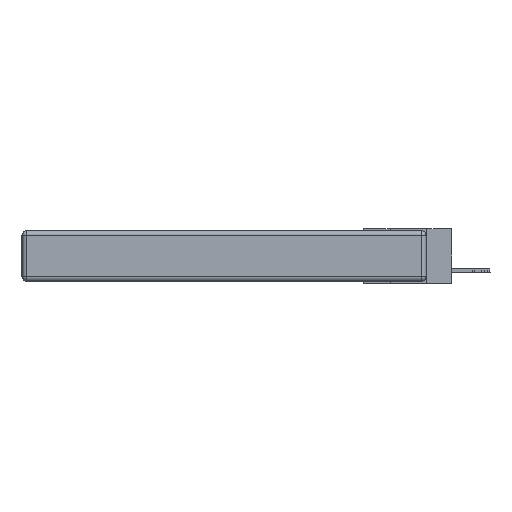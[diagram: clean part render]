
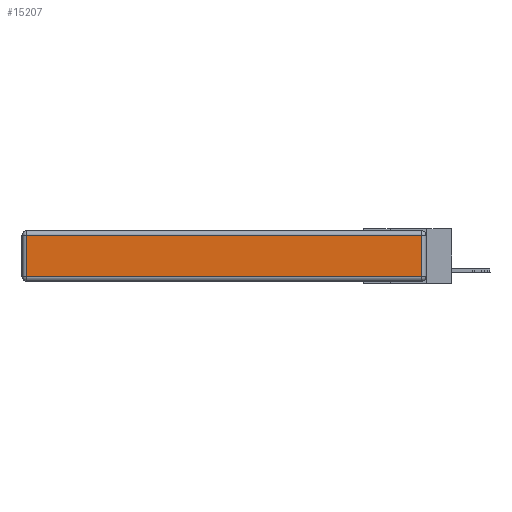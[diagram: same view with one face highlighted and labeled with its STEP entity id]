
A CAD part, left-side view. The second image highlights one B-rep face of the part: STEP entity #15207.
In plain terms, the highlighted planar face has unit normal (-1, 0, 0).
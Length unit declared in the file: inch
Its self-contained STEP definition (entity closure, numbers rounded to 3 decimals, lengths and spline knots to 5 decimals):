
#182 = ORIENTED_EDGE ( 'NONE', *, *, #19351, .T. ) ;
#227 = VERTEX_POINT ( 'NONE', #25936 ) ;
#235 = CARTESIAN_POINT ( 'NONE',  ( 0., 0.03, -0.343 ) ) ;
#1325 = PLANE ( 'NONE',  #10417 ) ;
#2420 = DIRECTION ( 'NONE',  ( 0., 0., 1. ) ) ;
#5226 = VECTOR ( 'NONE', #2420, 39.37008 ) ;
#6656 = DIRECTION ( 'NONE',  ( 0., 0., 1. ) ) ;
#8117 = CARTESIAN_POINT ( 'NONE',  ( 0., 0., -0.313 ) ) ;
#8878 = FACE_OUTER_BOUND ( 'NONE', #27182, .T. ) ;
#10362 = ORIENTED_EDGE ( 'NONE', *, *, #26238, .T. ) ;
#10417 = AXIS2_PLACEMENT_3D ( 'NONE', #11458, #18902, #6656 ) ;
#11458 = CARTESIAN_POINT ( 'NONE',  ( 0., 0., -0.343 ) ) ;
#12166 = VERTEX_POINT ( 'NONE', #22477 ) ;
#13234 = LINE ( 'NONE', #8117, #27146 ) ;
#13450 = VECTOR ( 'NONE', #22171, 39.37008 ) ;
#14374 = VECTOR ( 'NONE', #28630, 39.37008 ) ;
#15207 = ADVANCED_FACE ( 'NONE', ( #8878 ), #1325, .T. ) ;
#15752 = LINE ( 'NONE', #235, #5226 ) ;
#18863 = CARTESIAN_POINT ( 'NONE',  ( 0., 0.03, -0.313 ) ) ;
#18902 = DIRECTION ( 'NONE',  ( -1., 0., 0. ) ) ;
#19351 = EDGE_CURVE ( 'NONE', #31159, #12166, #20966, .T. ) ;
#20891 = CARTESIAN_POINT ( 'NONE',  ( 0., 2.72, -0.343 ) ) ;
#20966 = LINE ( 'NONE', #20891, #14374 ) ;
#21743 = EDGE_CURVE ( 'NONE', #22734, #227, #15752, .T. ) ;
#22171 = DIRECTION ( 'NONE',  ( 0., 1., 0. ) ) ;
#22279 = CARTESIAN_POINT ( 'NONE',  ( 0., 2.75, -0.03 ) ) ;
#22477 = CARTESIAN_POINT ( 'NONE',  ( 0., 2.72, -0.313 ) ) ;
#22580 = CARTESIAN_POINT ( 'NONE',  ( 0., 2.72, -0.03 ) ) ;
#22734 = VERTEX_POINT ( 'NONE', #18863 ) ;
#22747 = ORIENTED_EDGE ( 'NONE', *, *, #26642, .T. ) ;
#25341 = ORIENTED_EDGE ( 'NONE', *, *, #21743, .T. ) ;
#25459 = DIRECTION ( 'NONE',  ( 0., -1., 0. ) ) ;
#25936 = CARTESIAN_POINT ( 'NONE',  ( 0., 0.03, -0.03 ) ) ;
#26238 = EDGE_CURVE ( 'NONE', #227, #31159, #32107, .T. ) ;
#26642 = EDGE_CURVE ( 'NONE', #12166, #22734, #13234, .T. ) ;
#27146 = VECTOR ( 'NONE', #25459, 39.37008 ) ;
#27182 = EDGE_LOOP ( 'NONE', ( #22747, #25341, #10362, #182 ) ) ;
#28630 = DIRECTION ( 'NONE',  ( 0., 0., -1. ) ) ;
#31159 = VERTEX_POINT ( 'NONE', #22580 ) ;
#32107 = LINE ( 'NONE', #22279, #13450 ) ;
